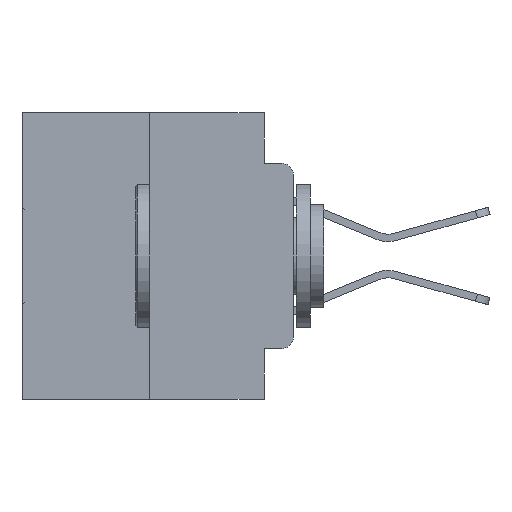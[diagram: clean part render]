
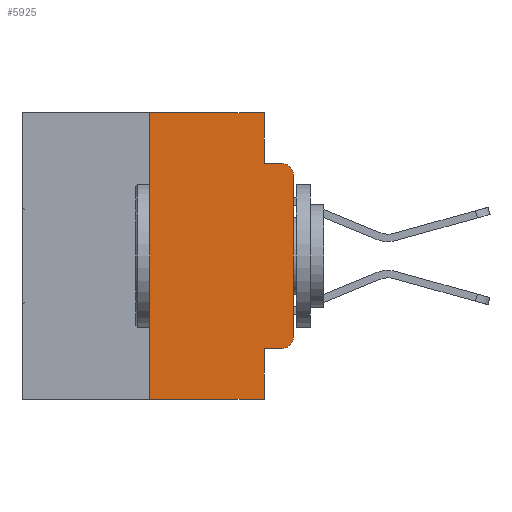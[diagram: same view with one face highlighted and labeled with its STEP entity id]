
A CAD part, left-side view. The second image highlights one B-rep face of the part: STEP entity #5925.
In plain terms, the highlighted planar face has unit normal (-1, 0, 0).
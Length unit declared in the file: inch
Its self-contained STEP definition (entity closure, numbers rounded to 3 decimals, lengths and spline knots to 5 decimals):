
#267 = CARTESIAN_POINT ( 'NONE',  ( 0., 0., 0. ) ) ;
#491 = ORIENTED_EDGE ( 'NONE', *, *, #1197, .F. ) ;
#826 = LINE ( 'NONE', #22517, #24994 ) ;
#1123 = PLANE ( 'NONE',  #24138 ) ;
#1197 = EDGE_CURVE ( 'NONE', #26343, #24493, #20239, .T. ) ;
#1754 = CARTESIAN_POINT ( 'NONE',  ( 0., 0.473, 0. ) ) ;
#2636 = DIRECTION ( 'NONE',  ( 0., 0., 1. ) ) ;
#2800 = EDGE_CURVE ( 'NONE', #10967, #26343, #826, .T. ) ;
#3474 = LINE ( 'NONE', #12560, #3524 ) ;
#3485 = CIRCLE ( 'NONE', #7488, 0.02 ) ;
#3521 = VECTOR ( 'NONE', #13338, 39.37008 ) ;
#3524 = VECTOR ( 'NONE', #14886, 39.37008 ) ;
#3567 = DIRECTION ( 'NONE',  ( 0., 0., -1. ) ) ;
#3816 = CARTESIAN_POINT ( 'NONE',  ( 0., 0.25, 0. ) ) ;
#4812 = DIRECTION ( 'NONE',  ( -1., 0., 0. ) ) ;
#5047 = ORIENTED_EDGE ( 'NONE', *, *, #14518, .F. ) ;
#5179 = CARTESIAN_POINT ( 'NONE',  ( 0., 0., -0.1085 ) ) ;
#5275 = VERTEX_POINT ( 'NONE', #16496 ) ;
#5446 = VECTOR ( 'NONE', #17732, 39.37008 ) ;
#5925 = ADVANCED_FACE ( 'NONE', ( #27679 ), #1123, .F. ) ;
#6594 = CARTESIAN_POINT ( 'NONE',  ( 0., 0., -0.3915 ) ) ;
#7007 = ORIENTED_EDGE ( 'NONE', *, *, #30222, .T. ) ;
#7488 = AXIS2_PLACEMENT_3D ( 'NONE', #19815, #24762, #22135 ) ;
#7516 = VECTOR ( 'NONE', #3567, 39.37008 ) ;
#7737 = VERTEX_POINT ( 'NONE', #18118 ) ;
#8052 = CARTESIAN_POINT ( 'NONE',  ( 0., 0.051, -0.0885 ) ) ;
#8288 = LINE ( 'NONE', #17788, #7516 ) ;
#9340 = VECTOR ( 'NONE', #19304, 39.37008 ) ;
#9657 = CARTESIAN_POINT ( 'NONE',  ( 0., 0.02, -0.3915 ) ) ;
#9964 = CARTESIAN_POINT ( 'NONE',  ( 0., 0.473, -0.5 ) ) ;
#10095 = CARTESIAN_POINT ( 'NONE',  ( 0., 0.02, -0.0885 ) ) ;
#10967 = VERTEX_POINT ( 'NONE', #14600 ) ;
#11072 = EDGE_CURVE ( 'NONE', #24493, #22820, #17417, .T. ) ;
#11180 = LINE ( 'NONE', #3816, #3521 ) ;
#11528 = VECTOR ( 'NONE', #29748, 39.37008 ) ;
#12560 = CARTESIAN_POINT ( 'NONE',  ( 0., 0.051, -0.4115 ) ) ;
#12582 = VERTEX_POINT ( 'NONE', #15849 ) ;
#12606 = EDGE_LOOP ( 'NONE', ( #16360, #7007, #26793, #491, #26670, #5047, #24878, #16536, #28377, #16687 ) ) ;
#12843 = EDGE_CURVE ( 'NONE', #27481, #7737, #3474, .T. ) ;
#13338 = DIRECTION ( 'NONE',  ( 0., 0., 1. ) ) ;
#13372 = VERTEX_POINT ( 'NONE', #5179 ) ;
#14518 = EDGE_CURVE ( 'NONE', #5275, #10967, #11180, .T. ) ;
#14600 = CARTESIAN_POINT ( 'NONE',  ( 0., 0.25, 0. ) ) ;
#14810 = CARTESIAN_POINT ( 'NONE',  ( 0., 0.051, -0.4115 ) ) ;
#14886 = DIRECTION ( 'NONE',  ( 0., -1., 0. ) ) ;
#15084 = VERTEX_POINT ( 'NONE', #6594 ) ;
#15659 = DIRECTION ( 'NONE',  ( 1., 0., 0. ) ) ;
#15849 = CARTESIAN_POINT ( 'NONE',  ( 0., 0.051, -0.5 ) ) ;
#16360 = ORIENTED_EDGE ( 'NONE', *, *, #28718, .T. ) ;
#16496 = CARTESIAN_POINT ( 'NONE',  ( 0., 0.25, -0.5 ) ) ;
#16536 = ORIENTED_EDGE ( 'NONE', *, *, #30577, .F. ) ;
#16687 = ORIENTED_EDGE ( 'NONE', *, *, #21487, .T. ) ;
#16694 = LINE ( 'NONE', #267, #22431 ) ;
#17417 = LINE ( 'NONE', #27084, #5446 ) ;
#17732 = DIRECTION ( 'NONE',  ( 0., -1., 0. ) ) ;
#17788 = CARTESIAN_POINT ( 'NONE',  ( 0., 0.051, 0. ) ) ;
#17859 = DIRECTION ( 'NONE',  ( 0., -1., 0. ) ) ;
#18118 = CARTESIAN_POINT ( 'NONE',  ( 0., 0.02, -0.4115 ) ) ;
#18305 = DIRECTION ( 'NONE',  ( 0., 0., -1. ) ) ;
#18642 = CARTESIAN_POINT ( 'NONE',  ( 0., 0.051, 0. ) ) ;
#19304 = DIRECTION ( 'NONE',  ( 0., -1., 0. ) ) ;
#19815 = CARTESIAN_POINT ( 'NONE',  ( 0., 0.02, -0.1085 ) ) ;
#20202 = CIRCLE ( 'NONE', #22672, 0.02 ) ;
#20239 = LINE ( 'NONE', #22555, #11528 ) ;
#21487 = EDGE_CURVE ( 'NONE', #7737, #15084, #20202, .T. ) ;
#22135 = DIRECTION ( 'NONE',  ( 0., 0., -1. ) ) ;
#22431 = VECTOR ( 'NONE', #2636, 39.37008 ) ;
#22517 = CARTESIAN_POINT ( 'NONE',  ( 0., 0.473, 0. ) ) ;
#22555 = CARTESIAN_POINT ( 'NONE',  ( 0., 0.051, 0. ) ) ;
#22672 = AXIS2_PLACEMENT_3D ( 'NONE', #9657, #4812, #25849 ) ;
#22820 = VERTEX_POINT ( 'NONE', #10095 ) ;
#23753 = EDGE_CURVE ( 'NONE', #5275, #12582, #26296, .T. ) ;
#24138 = AXIS2_PLACEMENT_3D ( 'NONE', #1754, #15659, #18305 ) ;
#24493 = VERTEX_POINT ( 'NONE', #8052 ) ;
#24762 = DIRECTION ( 'NONE',  ( -1., 0., 0. ) ) ;
#24878 = ORIENTED_EDGE ( 'NONE', *, *, #23753, .T. ) ;
#24994 = VECTOR ( 'NONE', #17859, 39.37008 ) ;
#25849 = DIRECTION ( 'NONE',  ( 0., 0., -1. ) ) ;
#26296 = LINE ( 'NONE', #9964, #9340 ) ;
#26343 = VERTEX_POINT ( 'NONE', #18642 ) ;
#26670 = ORIENTED_EDGE ( 'NONE', *, *, #2800, .F. ) ;
#26793 = ORIENTED_EDGE ( 'NONE', *, *, #11072, .F. ) ;
#27084 = CARTESIAN_POINT ( 'NONE',  ( 0., 0.051, -0.0885 ) ) ;
#27481 = VERTEX_POINT ( 'NONE', #14810 ) ;
#27679 = FACE_OUTER_BOUND ( 'NONE', #12606, .T. ) ;
#28377 = ORIENTED_EDGE ( 'NONE', *, *, #12843, .T. ) ;
#28718 = EDGE_CURVE ( 'NONE', #15084, #13372, #16694, .T. ) ;
#29748 = DIRECTION ( 'NONE',  ( 0., 0., -1. ) ) ;
#30222 = EDGE_CURVE ( 'NONE', #13372, #22820, #3485, .T. ) ;
#30577 = EDGE_CURVE ( 'NONE', #27481, #12582, #8288, .T. ) ;
